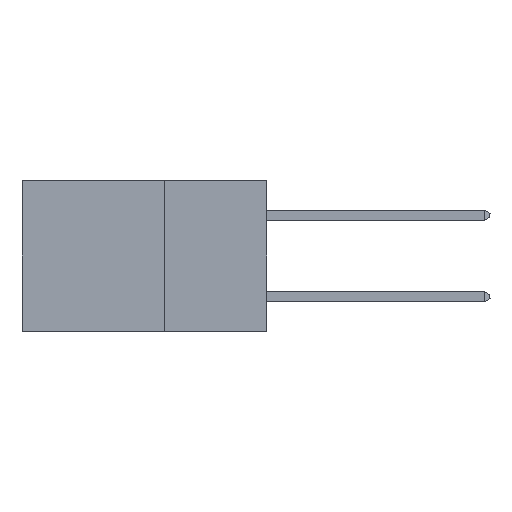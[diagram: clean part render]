
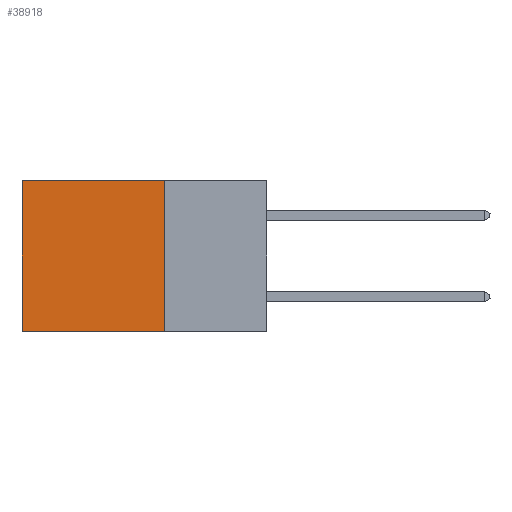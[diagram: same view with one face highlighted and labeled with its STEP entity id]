
A CAD part, left-side view. The second image highlights one B-rep face of the part: STEP entity #38918.
In plain terms, the highlighted planar face has unit normal (-1, 0, 0).
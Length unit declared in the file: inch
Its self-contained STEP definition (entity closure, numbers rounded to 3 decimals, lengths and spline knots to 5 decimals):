
#2042 = LINE ( 'NONE', #15628, #10512 ) ;
#4066 = PLANE ( 'NONE',  #5281 ) ;
#4527 = CARTESIAN_POINT ( 'NONE',  ( 0.2875, 0.25, 0. ) ) ;
#4786 = EDGE_CURVE ( 'NONE', #11773, #46105, #25131, .T. ) ;
#5281 = AXIS2_PLACEMENT_3D ( 'NONE', #4527, #25638, #36778 ) ;
#5418 = VECTOR ( 'NONE', #30535, 39.37008 ) ;
#5626 = LINE ( 'NONE', #39032, #11870 ) ;
#8101 = VERTEX_POINT ( 'NONE', #29846 ) ;
#9023 = VECTOR ( 'NONE', #40892, 39.37008 ) ;
#10512 = VECTOR ( 'NONE', #30051, 39.37008 ) ;
#11213 = ORIENTED_EDGE ( 'NONE', *, *, #12695, .F. ) ;
#11773 = VERTEX_POINT ( 'NONE', #31685 ) ;
#11870 = VECTOR ( 'NONE', #17553, 39.37008 ) ;
#12506 = ORIENTED_EDGE ( 'NONE', *, *, #4786, .T. ) ;
#12695 = EDGE_CURVE ( 'NONE', #8101, #17326, #2042, .T. ) ;
#15628 = CARTESIAN_POINT ( 'NONE',  ( 0.2875, 0.25, 0. ) ) ;
#17326 = VERTEX_POINT ( 'NONE', #40160 ) ;
#17553 = DIRECTION ( 'NONE',  ( 0., 1., 0. ) ) ;
#21946 = LINE ( 'NONE', #40735, #9023 ) ;
#25131 = LINE ( 'NONE', #34451, #5418 ) ;
#25638 = DIRECTION ( 'NONE',  ( 1., 0., 0. ) ) ;
#29846 = CARTESIAN_POINT ( 'NONE',  ( 0.2875, 0.25, 0. ) ) ;
#30051 = DIRECTION ( 'NONE',  ( 0., 0., -1. ) ) ;
#30142 = CARTESIAN_POINT ( 'NONE',  ( 0.2875, 0.6, -0.37 ) ) ;
#30535 = DIRECTION ( 'NONE',  ( 0., 0., -1. ) ) ;
#31685 = CARTESIAN_POINT ( 'NONE',  ( 0.2875, 0.6, 0. ) ) ;
#34451 = CARTESIAN_POINT ( 'NONE',  ( 0.2875, 0.6, 0. ) ) ;
#36778 = DIRECTION ( 'NONE',  ( 0., 0., -1. ) ) ;
#38918 = ADVANCED_FACE ( 'NONE', ( #43893 ), #4066, .F. ) ;
#39032 = CARTESIAN_POINT ( 'NONE',  ( 0.2875, 0.25, -0.37 ) ) ;
#40160 = CARTESIAN_POINT ( 'NONE',  ( 0.2875, 0.25, -0.37 ) ) ;
#40735 = CARTESIAN_POINT ( 'NONE',  ( 0.2875, 0.25, 0. ) ) ;
#40892 = DIRECTION ( 'NONE',  ( 0., 1., 0. ) ) ;
#42060 = EDGE_CURVE ( 'NONE', #8101, #11773, #21946, .T. ) ;
#43893 = FACE_OUTER_BOUND ( 'NONE', #45511, .T. ) ;
#44620 = EDGE_CURVE ( 'NONE', #17326, #46105, #5626, .T. ) ;
#44932 = ORIENTED_EDGE ( 'NONE', *, *, #44620, .F. ) ;
#45511 = EDGE_LOOP ( 'NONE', ( #12506, #44932, #11213, #46305 ) ) ;
#46105 = VERTEX_POINT ( 'NONE', #30142 ) ;
#46305 = ORIENTED_EDGE ( 'NONE', *, *, #42060, .T. ) ;
